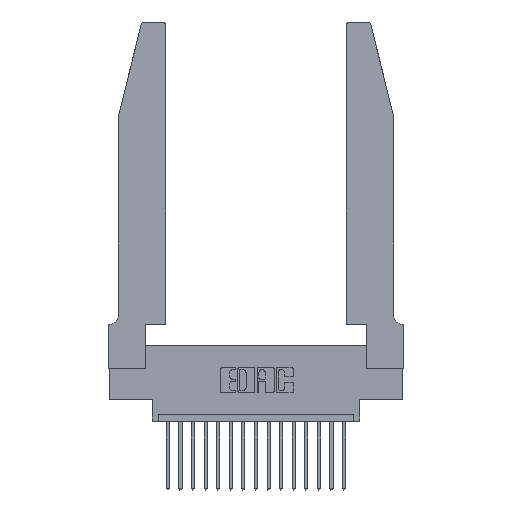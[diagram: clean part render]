
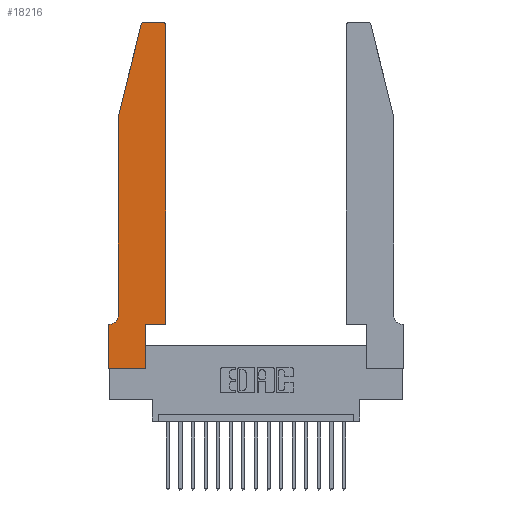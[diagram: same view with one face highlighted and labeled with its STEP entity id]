
A CAD part, top view. The second image highlights one B-rep face of the part: STEP entity #18216.
In plain terms, the highlighted planar face has unit normal (0, 0, 1).
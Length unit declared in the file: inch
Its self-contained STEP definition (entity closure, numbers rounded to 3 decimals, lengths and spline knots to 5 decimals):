
#81 = DIRECTION ( 'NONE',  ( 1., 0., 0. ) ) ;
#136 = ORIENTED_EDGE ( 'NONE', *, *, #12828, .T. ) ;
#174 = LINE ( 'NONE', #3374, #15919 ) ;
#257 = VECTOR ( 'NONE', #16288, 39.37008 ) ;
#280 = ORIENTED_EDGE ( 'NONE', *, *, #10012, .T. ) ;
#404 = DIRECTION ( 'NONE',  ( -1., 0., 0. ) ) ;
#407 = CARTESIAN_POINT ( 'NONE',  ( 0.25487, 2.72718, 0.37 ) ) ;
#706 = VERTEX_POINT ( 'NONE', #14843 ) ;
#890 = EDGE_CURVE ( 'NONE', #2143, #12415, #8999, .T. ) ;
#912 = CARTESIAN_POINT ( 'NONE',  ( 0.0755, 2., 0.37 ) ) ;
#957 = VECTOR ( 'NONE', #4711, 39.37008 ) ;
#1273 = AXIS2_PLACEMENT_3D ( 'NONE', #3210, #1794, #15787 ) ;
#1538 = ORIENTED_EDGE ( 'NONE', *, *, #8297, .T. ) ;
#1629 = EDGE_CURVE ( 'NONE', #18215, #2143, #19289, .T. ) ;
#1794 = DIRECTION ( 'NONE',  ( 0., 0., -1. ) ) ;
#2143 = VERTEX_POINT ( 'NONE', #407 ) ;
#2416 = VERTEX_POINT ( 'NONE', #18096 ) ;
#2658 = DIRECTION ( 'NONE',  ( 0., -1., 0. ) ) ;
#2687 = VERTEX_POINT ( 'NONE', #7440 ) ;
#2927 = VERTEX_POINT ( 'NONE', #18690 ) ;
#3210 = CARTESIAN_POINT ( 'NONE',  ( 0.0055, 0.42, 0.37 ) ) ;
#3232 = CARTESIAN_POINT ( 'NONE',  ( 0.4205, 2.75, 0.37 ) ) ;
#3374 = CARTESIAN_POINT ( 'NONE',  ( 0.2865, 0.35, 0.37 ) ) ;
#3979 = DIRECTION ( 'NONE',  ( -0.239, -0.971, 0. ) ) ;
#4164 = CARTESIAN_POINT ( 'NONE',  ( 0.284, 2.75, 0.37 ) ) ;
#4711 = DIRECTION ( 'NONE',  ( 1., 0., 0. ) ) ;
#4913 = EDGE_CURVE ( 'NONE', #2416, #18217, #6451, .T. ) ;
#4916 = VECTOR ( 'NONE', #7274, 39.37008 ) ;
#4930 = DIRECTION ( 'NONE',  ( 0., 0., 1. ) ) ;
#5093 = AXIS2_PLACEMENT_3D ( 'NONE', #5304, #8324, #19191 ) ;
#5184 = DIRECTION ( 'NONE',  ( 0., 1., 0. ) ) ;
#5304 = CARTESIAN_POINT ( 'NONE',  ( 0.4205, 2.72, 0.37 ) ) ;
#5321 = ORIENTED_EDGE ( 'NONE', *, *, #890, .T. ) ;
#5466 = FACE_OUTER_BOUND ( 'NONE', #9760, .T. ) ;
#5475 = DIRECTION ( 'NONE',  ( -1., 0., 0. ) ) ;
#5875 = VECTOR ( 'NONE', #3979, 39.37008 ) ;
#5994 = VERTEX_POINT ( 'NONE', #19391 ) ;
#6451 = LINE ( 'NONE', #7155, #17931 ) ;
#6669 = ORIENTED_EDGE ( 'NONE', *, *, #1629, .T. ) ;
#6736 = AXIS2_PLACEMENT_3D ( 'NONE', #15160, #13901, #81 ) ;
#6800 = DIRECTION ( 'NONE',  ( 1., 0., 0. ) ) ;
#6971 = EDGE_CURVE ( 'NONE', #9984, #706, #18827, .T. ) ;
#7155 = CARTESIAN_POINT ( 'NONE',  ( 0.0755, 0.35, 0.37 ) ) ;
#7274 = DIRECTION ( 'NONE',  ( 1., 0., 0. ) ) ;
#7440 = CARTESIAN_POINT ( 'NONE',  ( 0., 0., 0.37 ) ) ;
#7531 = CARTESIAN_POINT ( 'NONE',  ( 0., 0.35, 0.37 ) ) ;
#7534 = EDGE_CURVE ( 'NONE', #12415, #14953, #8245, .T. ) ;
#7902 = LINE ( 'NONE', #13855, #957 ) ;
#7959 = CARTESIAN_POINT ( 'NONE',  ( 0.2605, 2.75, 0.37 ) ) ;
#8245 = LINE ( 'NONE', #17769, #15618 ) ;
#8286 = CARTESIAN_POINT ( 'NONE',  ( 0.4505, 0.35, 0.37 ) ) ;
#8297 = EDGE_CURVE ( 'NONE', #706, #5994, #15867, .T. ) ;
#8324 = DIRECTION ( 'NONE',  ( 0., 0., 1. ) ) ;
#8999 = LINE ( 'NONE', #912, #5875 ) ;
#9243 = EDGE_CURVE ( 'NONE', #13960, #18215, #12530, .T. ) ;
#9253 = PLANE ( 'NONE',  #6736 ) ;
#9693 = ORIENTED_EDGE ( 'NONE', *, *, #11473, .T. ) ;
#9760 = EDGE_LOOP ( 'NONE', ( #11190, #6669, #5321, #10843, #9693, #14790, #16760, #11630, #136, #14998, #1538, #280 ) ) ;
#9984 = VERTEX_POINT ( 'NONE', #15838 ) ;
#10012 = EDGE_CURVE ( 'NONE', #5994, #13960, #19439, .T. ) ;
#10843 = ORIENTED_EDGE ( 'NONE', *, *, #7534, .T. ) ;
#11190 = ORIENTED_EDGE ( 'NONE', *, *, #9243, .T. ) ;
#11473 = EDGE_CURVE ( 'NONE', #14953, #2416, #14760, .T. ) ;
#11630 = ORIENTED_EDGE ( 'NONE', *, *, #17746, .T. ) ;
#11711 = CARTESIAN_POINT ( 'NONE',  ( 0., 0., 0.37 ) ) ;
#12415 = VERTEX_POINT ( 'NONE', #18504 ) ;
#12530 = LINE ( 'NONE', #7959, #17781 ) ;
#12828 = EDGE_CURVE ( 'NONE', #2927, #9984, #174, .T. ) ;
#13411 = LINE ( 'NONE', #11711, #257 ) ;
#13447 = AXIS2_PLACEMENT_3D ( 'NONE', #14072, #4930, #6800 ) ;
#13855 = CARTESIAN_POINT ( 'NONE',  ( 0., 0., 0.37 ) ) ;
#13901 = DIRECTION ( 'NONE',  ( 0., 0., 1. ) ) ;
#13960 = VERTEX_POINT ( 'NONE', #3232 ) ;
#14034 = DIRECTION ( 'NONE',  ( 0., 1., 0. ) ) ;
#14072 = CARTESIAN_POINT ( 'NONE',  ( 0.284, 2.72, 0.37 ) ) ;
#14760 = CIRCLE ( 'NONE', #1273, 0.07 ) ;
#14790 = ORIENTED_EDGE ( 'NONE', *, *, #4913, .T. ) ;
#14843 = CARTESIAN_POINT ( 'NONE',  ( 0.4505, 0.35, 0.37 ) ) ;
#14902 = CARTESIAN_POINT ( 'NONE',  ( 0.0755, 0.42, 0.37 ) ) ;
#14953 = VERTEX_POINT ( 'NONE', #14902 ) ;
#14998 = ORIENTED_EDGE ( 'NONE', *, *, #6971, .T. ) ;
#15160 = CARTESIAN_POINT ( 'NONE',  ( 0., 0.35, 0.37 ) ) ;
#15618 = VECTOR ( 'NONE', #2658, 39.37008 ) ;
#15787 = DIRECTION ( 'NONE',  ( -1., 0., 0. ) ) ;
#15838 = CARTESIAN_POINT ( 'NONE',  ( 0.2865, 0.35, 0.37 ) ) ;
#15867 = LINE ( 'NONE', #18728, #16107 ) ;
#15919 = VECTOR ( 'NONE', #14034, 39.37008 ) ;
#16107 = VECTOR ( 'NONE', #5184, 39.37008 ) ;
#16288 = DIRECTION ( 'NONE',  ( 0., -1., 0. ) ) ;
#16760 = ORIENTED_EDGE ( 'NONE', *, *, #17283, .T. ) ;
#17283 = EDGE_CURVE ( 'NONE', #18217, #2687, #13411, .T. ) ;
#17746 = EDGE_CURVE ( 'NONE', #2687, #2927, #7902, .T. ) ;
#17769 = CARTESIAN_POINT ( 'NONE',  ( 0.0755, 2., 0.37 ) ) ;
#17781 = VECTOR ( 'NONE', #404, 39.37008 ) ;
#17931 = VECTOR ( 'NONE', #5475, 39.37008 ) ;
#18096 = CARTESIAN_POINT ( 'NONE',  ( 0.0055, 0.35, 0.37 ) ) ;
#18215 = VERTEX_POINT ( 'NONE', #4164 ) ;
#18216 = ADVANCED_FACE ( 'NONE', ( #5466 ), #9253, .T. ) ;
#18217 = VERTEX_POINT ( 'NONE', #7531 ) ;
#18504 = CARTESIAN_POINT ( 'NONE',  ( 0.0755, 2., 0.37 ) ) ;
#18690 = CARTESIAN_POINT ( 'NONE',  ( 0.2865, 0., 0.37 ) ) ;
#18728 = CARTESIAN_POINT ( 'NONE',  ( 0.4505, 0.35, 0.37 ) ) ;
#18827 = LINE ( 'NONE', #8286, #4916 ) ;
#19191 = DIRECTION ( 'NONE',  ( 1., 0., 0. ) ) ;
#19289 = CIRCLE ( 'NONE', #13447, 0.03 ) ;
#19391 = CARTESIAN_POINT ( 'NONE',  ( 0.4505, 2.72, 0.37 ) ) ;
#19439 = CIRCLE ( 'NONE', #5093, 0.03 ) ;
